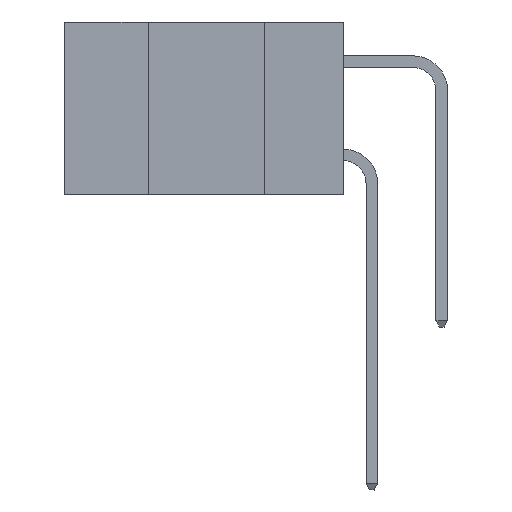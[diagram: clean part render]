
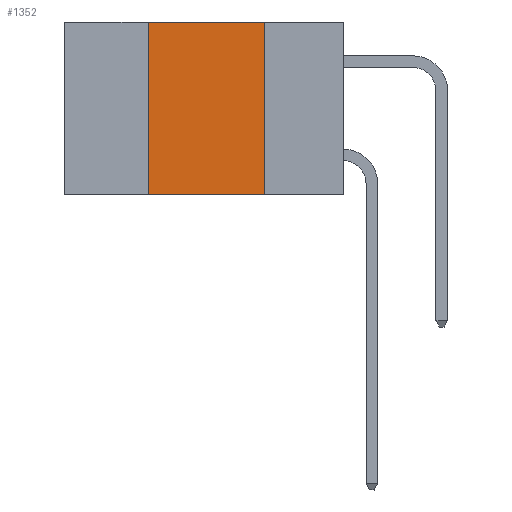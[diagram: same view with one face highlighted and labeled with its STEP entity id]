
A CAD part, left-side view. The second image highlights one B-rep face of the part: STEP entity #1352.
In plain terms, the highlighted planar face has unit normal (-1, 0, 0).
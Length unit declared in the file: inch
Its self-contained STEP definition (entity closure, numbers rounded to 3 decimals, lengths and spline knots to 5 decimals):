
#229 = PLANE ( 'NONE',  #10330 ) ;
#836 = VECTOR ( 'NONE', #9689, 39.37008 ) ;
#1195 = ORIENTED_EDGE ( 'NONE', *, *, #4014, .F. ) ;
#1352 = ADVANCED_FACE ( 'NONE', ( #4019 ), #229, .F. ) ;
#1712 = EDGE_CURVE ( 'NONE', #12069, #13130, #6970, .T. ) ;
#2021 = DIRECTION ( 'NONE',  ( 0., 0., -1. ) ) ;
#2428 = CARTESIAN_POINT ( 'NONE',  ( 0., 0.6, -0.37 ) ) ;
#2514 = LINE ( 'NONE', #5602, #836 ) ;
#2936 = DIRECTION ( 'NONE',  ( 0., 0., -1. ) ) ;
#4014 = EDGE_CURVE ( 'NONE', #8938, #9099, #8239, .T. ) ;
#4019 = FACE_OUTER_BOUND ( 'NONE', #10229, .T. ) ;
#4800 = ORIENTED_EDGE ( 'NONE', *, *, #6344, .T. ) ;
#5602 = CARTESIAN_POINT ( 'NONE',  ( 0., 0.6, 0. ) ) ;
#6319 = VECTOR ( 'NONE', #13172, 39.37008 ) ;
#6344 = EDGE_CURVE ( 'NONE', #8938, #13130, #6378, .T. ) ;
#6378 = LINE ( 'NONE', #2428, #12587 ) ;
#6970 = LINE ( 'NONE', #12924, #10336 ) ;
#7161 = CARTESIAN_POINT ( 'NONE',  ( 0., 0.42, -0.37 ) ) ;
#7387 = ORIENTED_EDGE ( 'NONE', *, *, #12267, .F. ) ;
#8193 = DIRECTION ( 'NONE',  ( 1., 0., 0. ) ) ;
#8239 = LINE ( 'NONE', #7161, #6319 ) ;
#8343 = ORIENTED_EDGE ( 'NONE', *, *, #1712, .F. ) ;
#8938 = VERTEX_POINT ( 'NONE', #12044 ) ;
#9099 = VERTEX_POINT ( 'NONE', #9255 ) ;
#9255 = CARTESIAN_POINT ( 'NONE',  ( 0., 0.42, 0. ) ) ;
#9316 = CARTESIAN_POINT ( 'NONE',  ( 0., 0.17, 0. ) ) ;
#9403 = CARTESIAN_POINT ( 'NONE',  ( 0., 0.6, 0. ) ) ;
#9689 = DIRECTION ( 'NONE',  ( 0., -1., 0. ) ) ;
#10229 = EDGE_LOOP ( 'NONE', ( #8343, #7387, #1195, #4800 ) ) ;
#10330 = AXIS2_PLACEMENT_3D ( 'NONE', #9403, #8193, #2021 ) ;
#10336 = VECTOR ( 'NONE', #2936, 39.37008 ) ;
#12044 = CARTESIAN_POINT ( 'NONE',  ( 0., 0.42, -0.37 ) ) ;
#12069 = VERTEX_POINT ( 'NONE', #9316 ) ;
#12267 = EDGE_CURVE ( 'NONE', #9099, #12069, #2514, .T. ) ;
#12297 = CARTESIAN_POINT ( 'NONE',  ( 0., 0.17, -0.37 ) ) ;
#12472 = DIRECTION ( 'NONE',  ( 0., -1., 0. ) ) ;
#12587 = VECTOR ( 'NONE', #12472, 39.37008 ) ;
#12924 = CARTESIAN_POINT ( 'NONE',  ( 0., 0.17, -0.37 ) ) ;
#13130 = VERTEX_POINT ( 'NONE', #12297 ) ;
#13172 = DIRECTION ( 'NONE',  ( 0., 0., 1. ) ) ;
